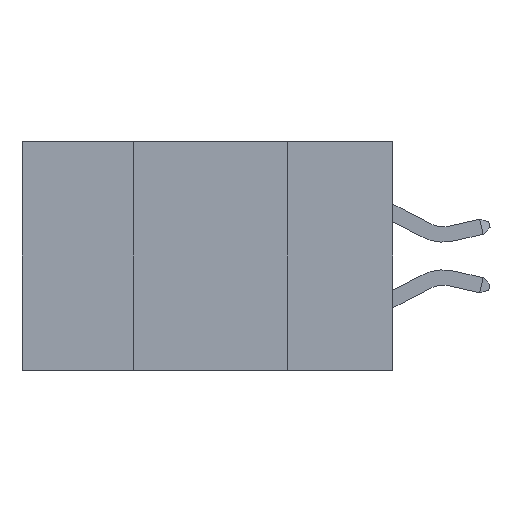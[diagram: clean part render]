
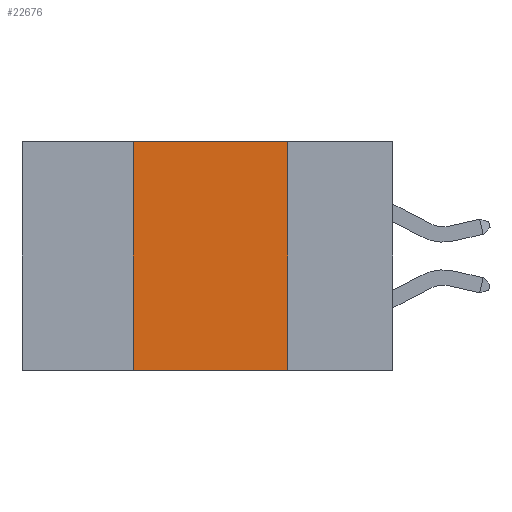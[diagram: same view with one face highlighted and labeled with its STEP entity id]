
A CAD part, left-side view. The second image highlights one B-rep face of the part: STEP entity #22676.
In plain terms, the highlighted planar face has unit normal (-1, 0, 0).
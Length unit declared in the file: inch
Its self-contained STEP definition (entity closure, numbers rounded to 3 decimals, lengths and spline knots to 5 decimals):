
#462 = VERTEX_POINT ( 'NONE', #16521 ) ;
#617 = CARTESIAN_POINT ( 'NONE',  ( 0., 0.42, 0. ) ) ;
#2283 = ORIENTED_EDGE ( 'NONE', *, *, #11571, .F. ) ;
#2755 = DIRECTION ( 'NONE',  ( 0., 0., 1. ) ) ;
#4874 = LINE ( 'NONE', #13529, #23260 ) ;
#6351 = PLANE ( 'NONE',  #16461 ) ;
#8211 = CARTESIAN_POINT ( 'NONE',  ( 0., 0.17, 0. ) ) ;
#8624 = FACE_OUTER_BOUND ( 'NONE', #35430, .T. ) ;
#10075 = VERTEX_POINT ( 'NONE', #24681 ) ;
#11230 = CARTESIAN_POINT ( 'NONE',  ( 0., 0.42, 0. ) ) ;
#11571 = EDGE_CURVE ( 'NONE', #17757, #10075, #20412, .T. ) ;
#12006 = DIRECTION ( 'NONE',  ( 1., 0., 0. ) ) ;
#13529 = CARTESIAN_POINT ( 'NONE',  ( 0., 0.6, -0.37 ) ) ;
#14459 = DIRECTION ( 'NONE',  ( 0., 0., -1. ) ) ;
#16273 = VECTOR ( 'NONE', #19871, 39.37008 ) ;
#16461 = AXIS2_PLACEMENT_3D ( 'NONE', #35013, #12006, #14459 ) ;
#16521 = CARTESIAN_POINT ( 'NONE',  ( 0., 0.42, -0.37 ) ) ;
#16691 = LINE ( 'NONE', #23056, #16273 ) ;
#16768 = EDGE_CURVE ( 'NONE', #462, #10075, #4874, .T. ) ;
#17757 = VERTEX_POINT ( 'NONE', #26276 ) ;
#19640 = DIRECTION ( 'NONE',  ( 0., 0., -1. ) ) ;
#19871 = DIRECTION ( 'NONE',  ( 0., -1., 0. ) ) ;
#20412 = LINE ( 'NONE', #8211, #25673 ) ;
#22105 = LINE ( 'NONE', #11230, #26299 ) ;
#22676 = ADVANCED_FACE ( 'NONE', ( #8624 ), #6351, .F. ) ;
#23056 = CARTESIAN_POINT ( 'NONE',  ( 0., 0.6, 0. ) ) ;
#23260 = VECTOR ( 'NONE', #28637, 39.37008 ) ;
#24681 = CARTESIAN_POINT ( 'NONE',  ( 0., 0.17, -0.37 ) ) ;
#25673 = VECTOR ( 'NONE', #19640, 39.37008 ) ;
#26276 = CARTESIAN_POINT ( 'NONE',  ( 0., 0.17, 0. ) ) ;
#26299 = VECTOR ( 'NONE', #2755, 39.37008 ) ;
#26657 = ORIENTED_EDGE ( 'NONE', *, *, #30055, .F. ) ;
#27742 = ORIENTED_EDGE ( 'NONE', *, *, #32920, .F. ) ;
#27880 = VERTEX_POINT ( 'NONE', #617 ) ;
#28637 = DIRECTION ( 'NONE',  ( 0., -1., 0. ) ) ;
#30055 = EDGE_CURVE ( 'NONE', #462, #27880, #22105, .T. ) ;
#32920 = EDGE_CURVE ( 'NONE', #27880, #17757, #16691, .T. ) ;
#35013 = CARTESIAN_POINT ( 'NONE',  ( 0., 0.6, 0. ) ) ;
#35430 = EDGE_LOOP ( 'NONE', ( #2283, #27742, #26657, #35531 ) ) ;
#35531 = ORIENTED_EDGE ( 'NONE', *, *, #16768, .T. ) ;
